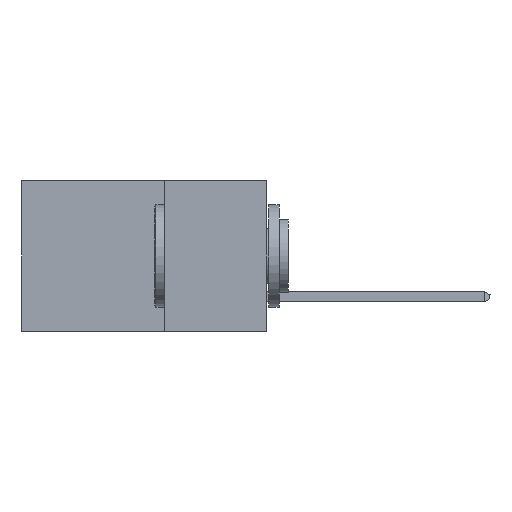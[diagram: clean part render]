
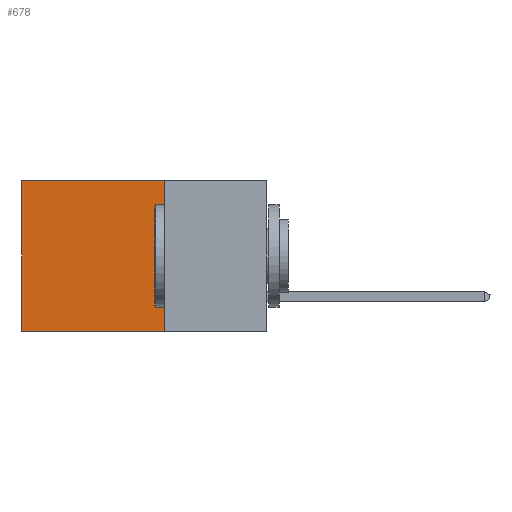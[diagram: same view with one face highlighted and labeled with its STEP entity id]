
A CAD part, left-side view. The second image highlights one B-rep face of the part: STEP entity #678.
In plain terms, the highlighted planar face has unit normal (-1, 0, 0).
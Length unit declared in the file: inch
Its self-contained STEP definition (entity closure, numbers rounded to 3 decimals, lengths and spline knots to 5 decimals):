
#678 = ADVANCED_FACE ( 'NONE', ( #32166 ), #9168, .F. ) ;
#2445 = CARTESIAN_POINT ( 'NONE',  ( 0.2875, 0.6, 0. ) ) ;
#3282 = VECTOR ( 'NONE', #12808, 39.37008 ) ;
#3347 = CARTESIAN_POINT ( 'NONE',  ( 0.2875, 0.6, -0.37 ) ) ;
#5330 = DIRECTION ( 'NONE',  ( 0., 0., -1. ) ) ;
#6319 = DIRECTION ( 'NONE',  ( 1., 0., 0. ) ) ;
#7324 = LINE ( 'NONE', #2445, #10464 ) ;
#8796 = DIRECTION ( 'NONE',  ( 0., 1., 0. ) ) ;
#9168 = PLANE ( 'NONE',  #31930 ) ;
#10101 = CARTESIAN_POINT ( 'NONE',  ( 0.2875, 0.25, 0. ) ) ;
#10193 = EDGE_LOOP ( 'NONE', ( #11203, #13452, #12529, #20892 ) ) ;
#10243 = VERTEX_POINT ( 'NONE', #19767 ) ;
#10464 = VECTOR ( 'NONE', #5330, 39.37008 ) ;
#10499 = EDGE_CURVE ( 'NONE', #23868, #10243, #14807, .T. ) ;
#11203 = ORIENTED_EDGE ( 'NONE', *, *, #23812, .T. ) ;
#12529 = ORIENTED_EDGE ( 'NONE', *, *, #10499, .F. ) ;
#12550 = CARTESIAN_POINT ( 'NONE',  ( 0.2875, 0.25, 0. ) ) ;
#12808 = DIRECTION ( 'NONE',  ( 0., 0., -1. ) ) ;
#13452 = ORIENTED_EDGE ( 'NONE', *, *, #35821, .F. ) ;
#13632 = VERTEX_POINT ( 'NONE', #19773 ) ;
#14807 = LINE ( 'NONE', #10101, #3282 ) ;
#16160 = VERTEX_POINT ( 'NONE', #3347 ) ;
#16593 = VECTOR ( 'NONE', #8796, 39.37008 ) ;
#19767 = CARTESIAN_POINT ( 'NONE',  ( 0.2875, 0.25, -0.37 ) ) ;
#19773 = CARTESIAN_POINT ( 'NONE',  ( 0.2875, 0.6, 0. ) ) ;
#20426 = CARTESIAN_POINT ( 'NONE',  ( 0.2875, 0.25, 0. ) ) ;
#20892 = ORIENTED_EDGE ( 'NONE', *, *, #32746, .T. ) ;
#22610 = CARTESIAN_POINT ( 'NONE',  ( 0.2875, 0.25, -0.37 ) ) ;
#23812 = EDGE_CURVE ( 'NONE', #13632, #16160, #7324, .T. ) ;
#23868 = VERTEX_POINT ( 'NONE', #12550 ) ;
#25126 = LINE ( 'NONE', #28076, #34426 ) ;
#26037 = DIRECTION ( 'NONE',  ( 0., 0., -1. ) ) ;
#28076 = CARTESIAN_POINT ( 'NONE',  ( 0.2875, 0.25, 0. ) ) ;
#28317 = DIRECTION ( 'NONE',  ( 0., 1., 0. ) ) ;
#28902 = LINE ( 'NONE', #22610, #16593 ) ;
#31930 = AXIS2_PLACEMENT_3D ( 'NONE', #20426, #6319, #26037 ) ;
#32166 = FACE_OUTER_BOUND ( 'NONE', #10193, .T. ) ;
#32746 = EDGE_CURVE ( 'NONE', #23868, #13632, #25126, .T. ) ;
#34426 = VECTOR ( 'NONE', #28317, 39.37008 ) ;
#35821 = EDGE_CURVE ( 'NONE', #10243, #16160, #28902, .T. ) ;
